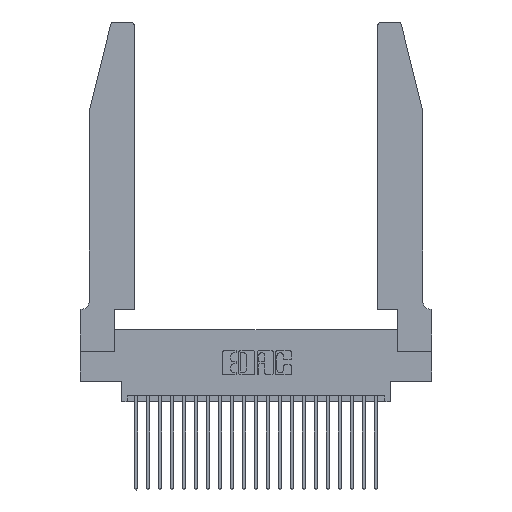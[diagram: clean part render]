
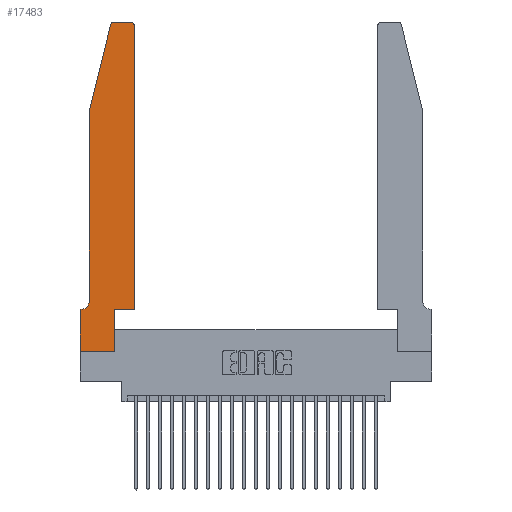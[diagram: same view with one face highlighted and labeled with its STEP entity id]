
A CAD part, top view. The second image highlights one B-rep face of the part: STEP entity #17483.
In plain terms, the highlighted planar face has unit normal (0, 0, 1).
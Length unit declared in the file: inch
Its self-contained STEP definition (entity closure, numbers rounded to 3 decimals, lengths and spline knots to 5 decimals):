
#29 = ORIENTED_EDGE ( 'NONE', *, *, #22308, .T. ) ;
#126 = VECTOR ( 'NONE', #21797, 39.37008 ) ;
#471 = CARTESIAN_POINT ( 'NONE',  ( 0.25487, 2.72718, 0.37 ) ) ;
#489 = EDGE_CURVE ( 'NONE', #20576, #13983, #23846, .T. ) ;
#493 = ORIENTED_EDGE ( 'NONE', *, *, #13987, .T. ) ;
#953 = VECTOR ( 'NONE', #15996, 39.37008 ) ;
#1110 = ORIENTED_EDGE ( 'NONE', *, *, #20009, .T. ) ;
#1128 = CARTESIAN_POINT ( 'NONE',  ( 0.4205, 2.72, 0.37 ) ) ;
#1195 = DIRECTION ( 'NONE',  ( 1., 0., 0. ) ) ;
#1921 = VECTOR ( 'NONE', #9892, 39.37008 ) ;
#2011 = CIRCLE ( 'NONE', #9284, 0.03 ) ;
#2107 = LINE ( 'NONE', #5968, #21397 ) ;
#2981 = CARTESIAN_POINT ( 'NONE',  ( 0.2865, 0.35, 0.37 ) ) ;
#3754 = CIRCLE ( 'NONE', #12019, 0.03 ) ;
#4533 = LINE ( 'NONE', #2981, #16791 ) ;
#4652 = CARTESIAN_POINT ( 'NONE',  ( 0.4505, 0.35, 0.37 ) ) ;
#4861 = ORIENTED_EDGE ( 'NONE', *, *, #10106, .T. ) ;
#5558 = VERTEX_POINT ( 'NONE', #15535 ) ;
#5968 = CARTESIAN_POINT ( 'NONE',  ( 0.0755, 0.35, 0.37 ) ) ;
#6016 = VERTEX_POINT ( 'NONE', #22537 ) ;
#6048 = EDGE_CURVE ( 'NONE', #18397, #5558, #2107, .T. ) ;
#6328 = CARTESIAN_POINT ( 'NONE',  ( 0.4505, 0.35, 0.37 ) ) ;
#6548 = CARTESIAN_POINT ( 'NONE',  ( 0.4505, 2.72, 0.37 ) ) ;
#6901 = DIRECTION ( 'NONE',  ( 0., 1., 0. ) ) ;
#6968 = CARTESIAN_POINT ( 'NONE',  ( 0.284, 2.72, 0.37 ) ) ;
#6988 = ORIENTED_EDGE ( 'NONE', *, *, #6048, .T. ) ;
#7487 = ORIENTED_EDGE ( 'NONE', *, *, #21239, .T. ) ;
#8145 = LINE ( 'NONE', #4652, #16280 ) ;
#8222 = EDGE_CURVE ( 'NONE', #13983, #6016, #3754, .T. ) ;
#8902 = DIRECTION ( 'NONE',  ( 1., 0., 0. ) ) ;
#9284 = AXIS2_PLACEMENT_3D ( 'NONE', #6968, #16046, #8902 ) ;
#9536 = EDGE_CURVE ( 'NONE', #18409, #12147, #4533, .T. ) ;
#9892 = DIRECTION ( 'NONE',  ( 0., 1., 0. ) ) ;
#9970 = CARTESIAN_POINT ( 'NONE',  ( 0., 0., 0.37 ) ) ;
#10106 = EDGE_CURVE ( 'NONE', #14092, #20051, #18540, .T. ) ;
#10216 = CARTESIAN_POINT ( 'NONE',  ( 0.4505, 0.35, 0.37 ) ) ;
#10248 = DIRECTION ( 'NONE',  ( -0.239, -0.971, 0. ) ) ;
#10262 = CARTESIAN_POINT ( 'NONE',  ( 0., 0.35, 0.37 ) ) ;
#10297 = CARTESIAN_POINT ( 'NONE',  ( 0.284, 2.75, 0.37 ) ) ;
#10603 = CARTESIAN_POINT ( 'NONE',  ( 0.0055, 0.35, 0.37 ) ) ;
#10633 = ORIENTED_EDGE ( 'NONE', *, *, #9536, .T. ) ;
#10964 = ORIENTED_EDGE ( 'NONE', *, *, #8222, .T. ) ;
#10976 = VECTOR ( 'NONE', #18015, 39.37008 ) ;
#12019 = AXIS2_PLACEMENT_3D ( 'NONE', #1128, #15853, #16019 ) ;
#12147 = VERTEX_POINT ( 'NONE', #15457 ) ;
#12211 = CARTESIAN_POINT ( 'NONE',  ( 0.0755, 2., 0.37 ) ) ;
#12232 = CARTESIAN_POINT ( 'NONE',  ( 0.0055, 0.42, 0.37 ) ) ;
#12708 = CARTESIAN_POINT ( 'NONE',  ( 0.0755, 0.42, 0.37 ) ) ;
#13204 = DIRECTION ( 'NONE',  ( -1., 0., 0. ) ) ;
#13469 = VERTEX_POINT ( 'NONE', #471 ) ;
#13560 = VECTOR ( 'NONE', #17693, 39.37008 ) ;
#13962 = EDGE_CURVE ( 'NONE', #12147, #20576, #8145, .T. ) ;
#13983 = VERTEX_POINT ( 'NONE', #6548 ) ;
#13987 = EDGE_CURVE ( 'NONE', #19221, #13469, #2011, .T. ) ;
#14092 = VERTEX_POINT ( 'NONE', #14106 ) ;
#14106 = CARTESIAN_POINT ( 'NONE',  ( 0.0755, 2., 0.37 ) ) ;
#14248 = FACE_OUTER_BOUND ( 'NONE', #16185, .T. ) ;
#14453 = LINE ( 'NONE', #21969, #126 ) ;
#15314 = PLANE ( 'NONE',  #22986 ) ;
#15457 = CARTESIAN_POINT ( 'NONE',  ( 0.2865, 0.35, 0.37 ) ) ;
#15520 = VECTOR ( 'NONE', #10248, 39.37008 ) ;
#15535 = CARTESIAN_POINT ( 'NONE',  ( 0., 0.35, 0.37 ) ) ;
#15853 = DIRECTION ( 'NONE',  ( 0., 0., 1. ) ) ;
#15933 = EDGE_CURVE ( 'NONE', #6016, #19221, #14453, .T. ) ;
#15996 = DIRECTION ( 'NONE',  ( 1., 0., 0. ) ) ;
#16019 = DIRECTION ( 'NONE',  ( 1., 0., 0. ) ) ;
#16046 = DIRECTION ( 'NONE',  ( 0., 0., 1. ) ) ;
#16185 = EDGE_LOOP ( 'NONE', ( #18354, #493, #17920, #4861, #7487, #6988, #1110, #29, #10633, #20645, #22612, #10964 ) ) ;
#16261 = VERTEX_POINT ( 'NONE', #9970 ) ;
#16280 = VECTOR ( 'NONE', #23154, 39.37008 ) ;
#16409 = CARTESIAN_POINT ( 'NONE',  ( 0.0755, 2., 0.37 ) ) ;
#16791 = VECTOR ( 'NONE', #6901, 39.37008 ) ;
#17483 = ADVANCED_FACE ( 'NONE', ( #14248 ), #15314, .T. ) ;
#17660 = LINE ( 'NONE', #21900, #10976 ) ;
#17693 = DIRECTION ( 'NONE',  ( 0., -1., 0. ) ) ;
#17713 = CARTESIAN_POINT ( 'NONE',  ( 0., 0., 0.37 ) ) ;
#17847 = DIRECTION ( 'NONE',  ( 0., 0., -1. ) ) ;
#17920 = ORIENTED_EDGE ( 'NONE', *, *, #21554, .T. ) ;
#18015 = DIRECTION ( 'NONE',  ( 0., -1., 0. ) ) ;
#18354 = ORIENTED_EDGE ( 'NONE', *, *, #15933, .T. ) ;
#18397 = VERTEX_POINT ( 'NONE', #10603 ) ;
#18409 = VERTEX_POINT ( 'NONE', #22575 ) ;
#18474 = CIRCLE ( 'NONE', #21111, 0.07 ) ;
#18540 = LINE ( 'NONE', #16409, #13560 ) ;
#19221 = VERTEX_POINT ( 'NONE', #10297 ) ;
#20009 = EDGE_CURVE ( 'NONE', #5558, #16261, #17660, .T. ) ;
#20051 = VERTEX_POINT ( 'NONE', #12708 ) ;
#20517 = LINE ( 'NONE', #12211, #15520 ) ;
#20576 = VERTEX_POINT ( 'NONE', #10216 ) ;
#20645 = ORIENTED_EDGE ( 'NONE', *, *, #13962, .T. ) ;
#21081 = LINE ( 'NONE', #17713, #953 ) ;
#21111 = AXIS2_PLACEMENT_3D ( 'NONE', #12232, #17847, #23556 ) ;
#21239 = EDGE_CURVE ( 'NONE', #20051, #18397, #18474, .T. ) ;
#21397 = VECTOR ( 'NONE', #13204, 39.37008 ) ;
#21554 = EDGE_CURVE ( 'NONE', #13469, #14092, #20517, .T. ) ;
#21797 = DIRECTION ( 'NONE',  ( -1., 0., 0. ) ) ;
#21900 = CARTESIAN_POINT ( 'NONE',  ( 0., 0., 0.37 ) ) ;
#21969 = CARTESIAN_POINT ( 'NONE',  ( 0.2605, 2.75, 0.37 ) ) ;
#22308 = EDGE_CURVE ( 'NONE', #16261, #18409, #21081, .T. ) ;
#22537 = CARTESIAN_POINT ( 'NONE',  ( 0.4205, 2.75, 0.37 ) ) ;
#22575 = CARTESIAN_POINT ( 'NONE',  ( 0.2865, 0., 0.37 ) ) ;
#22612 = ORIENTED_EDGE ( 'NONE', *, *, #489, .T. ) ;
#22943 = DIRECTION ( 'NONE',  ( 0., 0., 1. ) ) ;
#22986 = AXIS2_PLACEMENT_3D ( 'NONE', #10262, #22943, #1195 ) ;
#23154 = DIRECTION ( 'NONE',  ( 1., 0., 0. ) ) ;
#23556 = DIRECTION ( 'NONE',  ( -1., 0., 0. ) ) ;
#23846 = LINE ( 'NONE', #6328, #1921 ) ;
